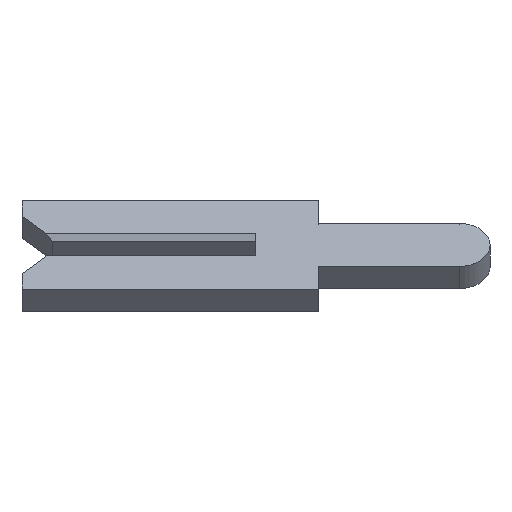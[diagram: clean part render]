
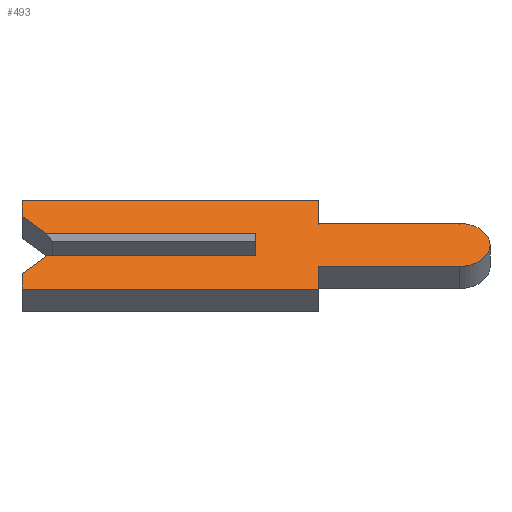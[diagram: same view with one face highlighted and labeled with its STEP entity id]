
A CAD part, left-side view. The second image highlights one B-rep face of the part: STEP entity #493.
In plain terms, the highlighted face is planar.
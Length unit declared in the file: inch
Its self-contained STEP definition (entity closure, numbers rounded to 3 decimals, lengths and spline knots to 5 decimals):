
#7 = CARTESIAN_POINT ( 'NONE',  ( -0.01, 0.15, -0.04 ) ) ;
#19 = PLANE ( 'NONE',  #366 ) ;
#31 = CARTESIAN_POINT ( 'NONE',  ( -0.01, -0.04, 0.0195 ) ) ;
#40 = VERTEX_POINT ( 'NONE', #837 ) ;
#67 = CIRCLE ( 'NONE', #472, 0.0195 ) ;
#76 = VERTEX_POINT ( 'NONE', #402 ) ;
#82 = ORIENTED_EDGE ( 'NONE', *, *, #537, .F. ) ;
#88 = EDGE_CURVE ( 'NONE', #331, #40, #67, .T. ) ;
#97 = DIRECTION ( 'NONE',  ( 0., 0., 1. ) ) ;
#105 = CARTESIAN_POINT ( 'NONE',  ( -0.01, 0.15, 0.04 ) ) ;
#108 = CARTESIAN_POINT ( 'NONE',  ( -0.01, 0.15, -0.04 ) ) ;
#115 = LINE ( 'NONE', #172, #470 ) ;
#126 = DIRECTION ( 'NONE',  ( 0., 0., -1. ) ) ;
#127 = VERTEX_POINT ( 'NONE', #624 ) ;
#132 = VECTOR ( 'NONE', #161, 39.37008 ) ;
#140 = CARTESIAN_POINT ( 'NONE',  ( -0.01, -0.1305, -0.01 ) ) ;
#152 = ORIENTED_EDGE ( 'NONE', *, *, #690, .F. ) ;
#154 = CARTESIAN_POINT ( 'NONE',  ( -0.01, -0.04, -0.0195 ) ) ;
#156 = CARTESIAN_POINT ( 'NONE',  ( -0.01, 0.1305, 0.0065 ) ) ;
#161 = DIRECTION ( 'NONE',  ( 0., 1., 0. ) ) ;
#168 = EDGE_CURVE ( 'NONE', #76, #743, #429, .T. ) ;
#172 = CARTESIAN_POINT ( 'NONE',  ( -0.01, 0.1305, -0.0065 ) ) ;
#173 = VERTEX_POINT ( 'NONE', #565 ) ;
#194 = VERTEX_POINT ( 'NONE', #277 ) ;
#199 = VECTOR ( 'NONE', #897, 39.37008 ) ;
#226 = EDGE_CURVE ( 'NONE', #173, #307, #724, .T. ) ;
#232 = LINE ( 'NONE', #156, #454 ) ;
#234 = ORIENTED_EDGE ( 'NONE', *, *, #588, .F. ) ;
#242 = VECTOR ( 'NONE', #500, 39.37008 ) ;
#249 = ORIENTED_EDGE ( 'NONE', *, *, #850, .F. ) ;
#256 = LINE ( 'NONE', #108, #199 ) ;
#277 = CARTESIAN_POINT ( 'NONE',  ( -0.01, 0.15, 0.026 ) ) ;
#278 = LINE ( 'NONE', #739, #835 ) ;
#282 = VERTEX_POINT ( 'NONE', #488 ) ;
#300 = VERTEX_POINT ( 'NONE', #371 ) ;
#307 = VERTEX_POINT ( 'NONE', #716 ) ;
#318 = ORIENTED_EDGE ( 'NONE', *, *, #226, .F. ) ;
#331 = VERTEX_POINT ( 'NONE', #871 ) ;
#366 = AXIS2_PLACEMENT_3D ( 'NONE', #526, #806, #726 ) ;
#371 = CARTESIAN_POINT ( 'NONE',  ( -0.01, 0.134, -0.01 ) ) ;
#388 = VERTEX_POINT ( 'NONE', #7 ) ;
#402 = CARTESIAN_POINT ( 'NONE',  ( -0.01, -0.04, 0.04 ) ) ;
#417 = VERTEX_POINT ( 'NONE', #647 ) ;
#429 = LINE ( 'NONE', #554, #242 ) ;
#432 = VECTOR ( 'NONE', #605, 39.37008 ) ;
#435 = ORIENTED_EDGE ( 'NONE', *, *, #168, .F. ) ;
#440 = LINE ( 'NONE', #665, #718 ) ;
#443 = DIRECTION ( 'NONE',  ( 0., 0.707, 0.707 ) ) ;
#449 = DIRECTION ( 'NONE',  ( 0., 0., -1. ) ) ;
#452 = VECTOR ( 'NONE', #597, 39.37008 ) ;
#453 = CARTESIAN_POINT ( 'NONE',  ( -0.01, -0.04, -0.04 ) ) ;
#454 = VECTOR ( 'NONE', #443, 39.37008 ) ;
#459 = CARTESIAN_POINT ( 'NONE',  ( -0.01, -0.04, 0.0195 ) ) ;
#470 = VECTOR ( 'NONE', #822, 39.37008 ) ;
#472 = AXIS2_PLACEMENT_3D ( 'NONE', #681, #754, #126 ) ;
#483 = LINE ( 'NONE', #105, #552 ) ;
#484 = EDGE_CURVE ( 'NONE', #300, #173, #729, .T. ) ;
#488 = CARTESIAN_POINT ( 'NONE',  ( -0.01, 0.134, 0.01 ) ) ;
#493 = ADVANCED_FACE ( 'NONE', ( #582 ), #19, .F. ) ;
#500 = DIRECTION ( 'NONE',  ( 0., 0., -1. ) ) ;
#505 = DIRECTION ( 'NONE',  ( 0., -1., 0. ) ) ;
#526 = CARTESIAN_POINT ( 'NONE',  ( -0.01, -0.1305, 0. ) ) ;
#533 = ORIENTED_EDGE ( 'NONE', *, *, #615, .F. ) ;
#537 = EDGE_CURVE ( 'NONE', #40, #863, #888, .T. ) ;
#540 = VECTOR ( 'NONE', #505, 39.37008 ) ;
#552 = VECTOR ( 'NONE', #599, 39.37008 ) ;
#554 = CARTESIAN_POINT ( 'NONE',  ( -0.01, -0.04, 0.04 ) ) ;
#557 = ORIENTED_EDGE ( 'NONE', *, *, #88, .F. ) ;
#565 = CARTESIAN_POINT ( 'NONE',  ( -0.01, 0., -0.01 ) ) ;
#582 = FACE_OUTER_BOUND ( 'NONE', #886, .T. ) ;
#583 = EDGE_CURVE ( 'NONE', #863, #667, #744, .T. ) ;
#587 = CARTESIAN_POINT ( 'NONE',  ( -0.01, -0.04, -0.04 ) ) ;
#588 = EDGE_CURVE ( 'NONE', #282, #194, #232, .T. ) ;
#597 = DIRECTION ( 'NONE',  ( 0., -1., 0. ) ) ;
#599 = DIRECTION ( 'NONE',  ( 0., -1., 0. ) ) ;
#605 = DIRECTION ( 'NONE',  ( 0., -1., 0. ) ) ;
#615 = EDGE_CURVE ( 'NONE', #388, #417, #440, .T. ) ;
#617 = ORIENTED_EDGE ( 'NONE', *, *, #778, .F. ) ;
#624 = CARTESIAN_POINT ( 'NONE',  ( -0.01, 0.15, 0.04 ) ) ;
#640 = DIRECTION ( 'NONE',  ( 0., 0., 1. ) ) ;
#647 = CARTESIAN_POINT ( 'NONE',  ( -0.01, 0.15, -0.026 ) ) ;
#648 = ORIENTED_EDGE ( 'NONE', *, *, #796, .F. ) ;
#665 = CARTESIAN_POINT ( 'NONE',  ( -0.01, 0.15, -0.026 ) ) ;
#666 = DIRECTION ( 'NONE',  ( 0., 0., 1. ) ) ;
#667 = VERTEX_POINT ( 'NONE', #453 ) ;
#681 = CARTESIAN_POINT ( 'NONE',  ( -0.01, -0.1305, 0. ) ) ;
#690 = EDGE_CURVE ( 'NONE', #127, #76, #483, .T. ) ;
#692 = ORIENTED_EDGE ( 'NONE', *, *, #583, .F. ) ;
#716 = CARTESIAN_POINT ( 'NONE',  ( -0.01, 0., 0.01 ) ) ;
#718 = VECTOR ( 'NONE', #666, 39.37008 ) ;
#724 = LINE ( 'NONE', #849, #918 ) ;
#726 = DIRECTION ( 'NONE',  ( 0., 0., -1. ) ) ;
#729 = LINE ( 'NONE', #140, #540 ) ;
#739 = CARTESIAN_POINT ( 'NONE',  ( -0.01, 0.15, 0.026 ) ) ;
#743 = VERTEX_POINT ( 'NONE', #31 ) ;
#744 = LINE ( 'NONE', #587, #791 ) ;
#747 = CARTESIAN_POINT ( 'NONE',  ( -0.01, 0.15, 0.01 ) ) ;
#754 = DIRECTION ( 'NONE',  ( 1., 0., 0. ) ) ;
#778 = EDGE_CURVE ( 'NONE', #194, #127, #278, .T. ) ;
#781 = ORIENTED_EDGE ( 'NONE', *, *, #825, .F. ) ;
#791 = VECTOR ( 'NONE', #449, 39.37008 ) ;
#796 = EDGE_CURVE ( 'NONE', #417, #300, #115, .T. ) ;
#806 = DIRECTION ( 'NONE',  ( 1., 0., 0. ) ) ;
#820 = LINE ( 'NONE', #747, #432 ) ;
#821 = CARTESIAN_POINT ( 'NONE',  ( -0.01, -0.04, -0.0195 ) ) ;
#822 = DIRECTION ( 'NONE',  ( 0., -0.707, 0.707 ) ) ;
#825 = EDGE_CURVE ( 'NONE', #743, #331, #872, .T. ) ;
#835 = VECTOR ( 'NONE', #97, 39.37008 ) ;
#837 = CARTESIAN_POINT ( 'NONE',  ( -0.01, -0.1305, -0.0195 ) ) ;
#849 = CARTESIAN_POINT ( 'NONE',  ( -0.01, 0., 0.0065 ) ) ;
#850 = EDGE_CURVE ( 'NONE', #667, #388, #256, .T. ) ;
#863 = VERTEX_POINT ( 'NONE', #821 ) ;
#871 = CARTESIAN_POINT ( 'NONE',  ( -0.01, -0.1305, 0.0195 ) ) ;
#872 = LINE ( 'NONE', #459, #452 ) ;
#874 = ORIENTED_EDGE ( 'NONE', *, *, #880, .T. ) ;
#880 = EDGE_CURVE ( 'NONE', #282, #307, #820, .T. ) ;
#884 = ORIENTED_EDGE ( 'NONE', *, *, #484, .F. ) ;
#886 = EDGE_LOOP ( 'NONE', ( #874, #318, #884, #648, #533, #249, #692, #82, #557, #781, #435, #152, #617, #234 ) ) ;
#888 = LINE ( 'NONE', #154, #132 ) ;
#897 = DIRECTION ( 'NONE',  ( 0., 1., 0. ) ) ;
#918 = VECTOR ( 'NONE', #640, 39.37008 ) ;
